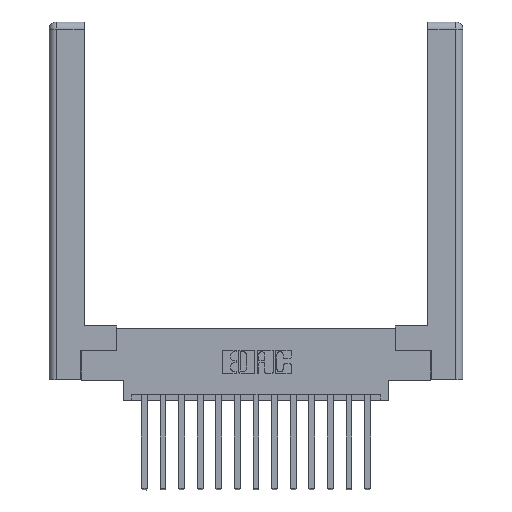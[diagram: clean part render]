
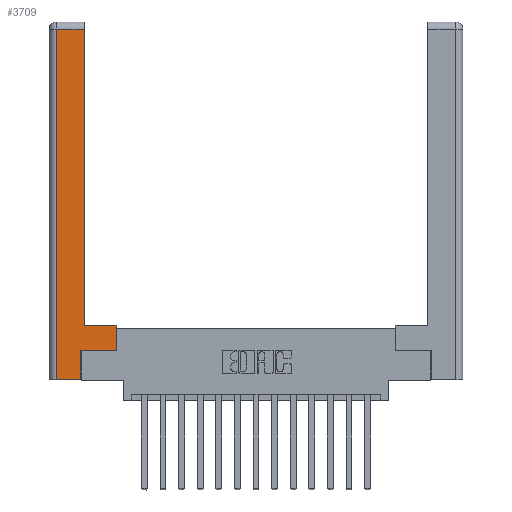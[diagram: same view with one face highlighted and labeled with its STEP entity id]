
A CAD part, top view. The second image highlights one B-rep face of the part: STEP entity #3709.
In plain terms, the highlighted planar face has unit normal (0, 0, 1).
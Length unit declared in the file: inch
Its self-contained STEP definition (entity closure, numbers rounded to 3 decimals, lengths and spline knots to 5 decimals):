
#9 = VERTEX_POINT ( 'NONE', #8457 ) ;
#307 = LINE ( 'NONE', #13835, #13427 ) ;
#376 = VERTEX_POINT ( 'NONE', #794 ) ;
#621 = EDGE_CURVE ( 'NONE', #9, #16305, #6227, .T. ) ;
#707 = DIRECTION ( 'NONE',  ( 1., 0., 0. ) ) ;
#743 = ORIENTED_EDGE ( 'NONE', *, *, #11676, .T. ) ;
#794 = CARTESIAN_POINT ( 'NONE',  ( 0.265, 0., 0. ) ) ;
#818 = CARTESIAN_POINT ( 'NONE',  ( 0.265, 0., 0. ) ) ;
#878 = DIRECTION ( 'NONE',  ( 1., 0., 0. ) ) ;
#1106 = VERTEX_POINT ( 'NONE', #13719 ) ;
#1262 = CARTESIAN_POINT ( 'NONE',  ( 0.295, 3., 0. ) ) ;
#1302 = ORIENTED_EDGE ( 'NONE', *, *, #16339, .T. ) ;
#1648 = ORIENTED_EDGE ( 'NONE', *, *, #14023, .T. ) ;
#2047 = DIRECTION ( 'NONE',  ( -1., 0., 0. ) ) ;
#2103 = CARTESIAN_POINT ( 'NONE',  ( 0.565, 0.245, 0. ) ) ;
#2234 = EDGE_CURVE ( 'NONE', #4404, #14991, #11329, .T. ) ;
#2491 = DIRECTION ( 'NONE',  ( 0., 1., 0. ) ) ;
#2630 = VERTEX_POINT ( 'NONE', #14906 ) ;
#3458 = CARTESIAN_POINT ( 'NONE',  ( 0.265, 0.245, 0. ) ) ;
#3602 = AXIS2_PLACEMENT_3D ( 'NONE', #3707, #10206, #8882 ) ;
#3645 = PLANE ( 'NONE',  #3602 ) ;
#3707 = CARTESIAN_POINT ( 'NONE',  ( 0., 0., 0. ) ) ;
#3709 = ADVANCED_FACE ( 'NONE', ( #8893 ), #3645, .F. ) ;
#3818 = ORIENTED_EDGE ( 'NONE', *, *, #7392, .T. ) ;
#3917 = ORIENTED_EDGE ( 'NONE', *, *, #2234, .T. ) ;
#4404 = VERTEX_POINT ( 'NONE', #15697 ) ;
#5108 = ORIENTED_EDGE ( 'NONE', *, *, #7458, .T. ) ;
#5587 = VECTOR ( 'NONE', #878, 39.37008 ) ;
#6227 = LINE ( 'NONE', #1262, #10593 ) ;
#6256 = CARTESIAN_POINT ( 'NONE',  ( 0.565, 0.45, 0. ) ) ;
#6346 = VECTOR ( 'NONE', #2047, 39.37008 ) ;
#7392 = EDGE_CURVE ( 'NONE', #2630, #376, #15282, .T. ) ;
#7458 = EDGE_CURVE ( 'NONE', #1106, #9, #11507, .T. ) ;
#7764 = EDGE_LOOP ( 'NONE', ( #13750, #743, #15660, #3818, #1648, #3917, #1302, #5108 ) ) ;
#8457 = CARTESIAN_POINT ( 'NONE',  ( 0.295, 0.45, 0. ) ) ;
#8722 = CARTESIAN_POINT ( 'NONE',  ( 0.0615, 2.94, 0. ) ) ;
#8882 = DIRECTION ( 'NONE',  ( -1., 0., 0. ) ) ;
#8893 = FACE_OUTER_BOUND ( 'NONE', #7764, .T. ) ;
#9260 = VECTOR ( 'NONE', #14936, 39.37008 ) ;
#9386 = LINE ( 'NONE', #8722, #9979 ) ;
#9620 = VERTEX_POINT ( 'NONE', #15310 ) ;
#9630 = CARTESIAN_POINT ( 'NONE',  ( 0.295, 0.45, 0. ) ) ;
#9979 = VECTOR ( 'NONE', #16230, 39.37008 ) ;
#10062 = LINE ( 'NONE', #3458, #9260 ) ;
#10130 = VECTOR ( 'NONE', #707, 39.37008 ) ;
#10206 = DIRECTION ( 'NONE',  ( 0., 0., -1. ) ) ;
#10593 = VECTOR ( 'NONE', #2491, 39.37008 ) ;
#11329 = LINE ( 'NONE', #2103, #5587 ) ;
#11507 = LINE ( 'NONE', #9630, #6346 ) ;
#11629 = CARTESIAN_POINT ( 'NONE',  ( 0.565, 0.245, 0. ) ) ;
#11676 = EDGE_CURVE ( 'NONE', #16305, #9620, #9386, .T. ) ;
#11697 = VECTOR ( 'NONE', #16423, 39.37008 ) ;
#12495 = CARTESIAN_POINT ( 'NONE',  ( 0.295, 2.94, 0. ) ) ;
#13427 = VECTOR ( 'NONE', #13782, 39.37008 ) ;
#13719 = CARTESIAN_POINT ( 'NONE',  ( 0.565, 0.45, 0. ) ) ;
#13750 = ORIENTED_EDGE ( 'NONE', *, *, #621, .T. ) ;
#13782 = DIRECTION ( 'NONE',  ( 0., -1., 0. ) ) ;
#13835 = CARTESIAN_POINT ( 'NONE',  ( 0.0615, 0., 0. ) ) ;
#14023 = EDGE_CURVE ( 'NONE', #376, #4404, #10062, .T. ) ;
#14803 = EDGE_CURVE ( 'NONE', #9620, #2630, #307, .T. ) ;
#14906 = CARTESIAN_POINT ( 'NONE',  ( 0.0615, 0., 0. ) ) ;
#14936 = DIRECTION ( 'NONE',  ( 0., 1., 0. ) ) ;
#14991 = VERTEX_POINT ( 'NONE', #11629 ) ;
#15089 = LINE ( 'NONE', #6256, #11697 ) ;
#15282 = LINE ( 'NONE', #818, #10130 ) ;
#15310 = CARTESIAN_POINT ( 'NONE',  ( 0.0615, 2.94, 0. ) ) ;
#15660 = ORIENTED_EDGE ( 'NONE', *, *, #14803, .T. ) ;
#15697 = CARTESIAN_POINT ( 'NONE',  ( 0.265, 0.245, 0. ) ) ;
#16230 = DIRECTION ( 'NONE',  ( -1., 0., 0. ) ) ;
#16305 = VERTEX_POINT ( 'NONE', #12495 ) ;
#16339 = EDGE_CURVE ( 'NONE', #14991, #1106, #15089, .T. ) ;
#16423 = DIRECTION ( 'NONE',  ( 0., 1., 0. ) ) ;
